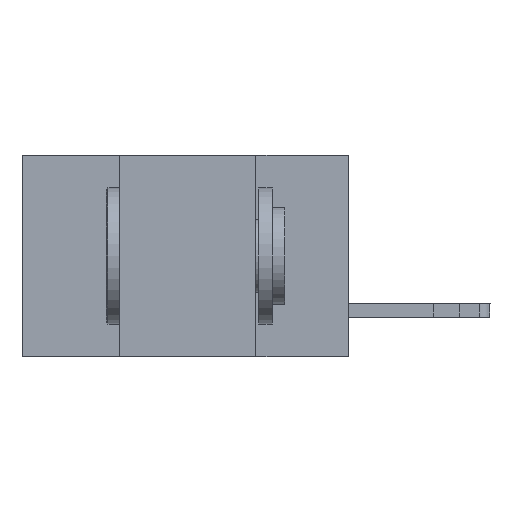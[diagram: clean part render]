
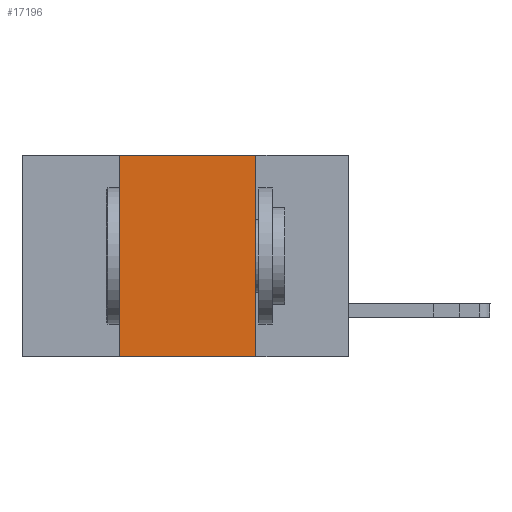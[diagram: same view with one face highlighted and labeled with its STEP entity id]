
A CAD part, left-side view. The second image highlights one B-rep face of the part: STEP entity #17196.
In plain terms, the highlighted planar face has unit normal (-1, 0, 0).
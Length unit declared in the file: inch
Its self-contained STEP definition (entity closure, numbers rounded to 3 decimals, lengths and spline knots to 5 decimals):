
#96 = CARTESIAN_POINT ( 'NONE',  ( 0., 0.6, -0.37 ) ) ;
#472 = CARTESIAN_POINT ( 'NONE',  ( 0., 0.42, -0.37 ) ) ;
#1150 = ORIENTED_EDGE ( 'NONE', *, *, #3767, .F. ) ;
#1240 = DIRECTION ( 'NONE',  ( 0., 0., 1. ) ) ;
#1275 = DIRECTION ( 'NONE',  ( 0., 0., -1. ) ) ;
#2081 = VERTEX_POINT ( 'NONE', #8609 ) ;
#2252 = ORIENTED_EDGE ( 'NONE', *, *, #8437, .F. ) ;
#2761 = CARTESIAN_POINT ( 'NONE',  ( 0., 0.42, -0.37 ) ) ;
#2810 = DIRECTION ( 'NONE',  ( 0., -1., 0. ) ) ;
#2941 = ORIENTED_EDGE ( 'NONE', *, *, #15125, .T. ) ;
#3767 = EDGE_CURVE ( 'NONE', #4106, #5642, #17734, .T. ) ;
#4106 = VERTEX_POINT ( 'NONE', #2761 ) ;
#4689 = EDGE_CURVE ( 'NONE', #5642, #8447, #13303, .T. ) ;
#5642 = VERTEX_POINT ( 'NONE', #7934 ) ;
#5670 = EDGE_LOOP ( 'NONE', ( #2252, #6712, #1150, #2941 ) ) ;
#6530 = LINE ( 'NONE', #96, #13383 ) ;
#6712 = ORIENTED_EDGE ( 'NONE', *, *, #4689, .F. ) ;
#7934 = CARTESIAN_POINT ( 'NONE',  ( 0., 0.42, 0. ) ) ;
#8136 = DIRECTION ( 'NONE',  ( 1., 0., 0. ) ) ;
#8437 = EDGE_CURVE ( 'NONE', #8447, #2081, #11788, .T. ) ;
#8447 = VERTEX_POINT ( 'NONE', #16274 ) ;
#8609 = CARTESIAN_POINT ( 'NONE',  ( 0., 0.17, -0.37 ) ) ;
#9552 = CARTESIAN_POINT ( 'NONE',  ( 0., 0.17, -0.37 ) ) ;
#11788 = LINE ( 'NONE', #9552, #14963 ) ;
#12199 = PLANE ( 'NONE',  #15303 ) ;
#12934 = FACE_OUTER_BOUND ( 'NONE', #5670, .T. ) ;
#13303 = LINE ( 'NONE', #13330, #16847 ) ;
#13330 = CARTESIAN_POINT ( 'NONE',  ( 0., 0.6, 0. ) ) ;
#13383 = VECTOR ( 'NONE', #2810, 39.37008 ) ;
#13560 = CARTESIAN_POINT ( 'NONE',  ( 0., 0.6, 0. ) ) ;
#13725 = DIRECTION ( 'NONE',  ( 0., -1., 0. ) ) ;
#14963 = VECTOR ( 'NONE', #1275, 39.37008 ) ;
#15125 = EDGE_CURVE ( 'NONE', #4106, #2081, #6530, .T. ) ;
#15303 = AXIS2_PLACEMENT_3D ( 'NONE', #13560, #8136, #17587 ) ;
#16274 = CARTESIAN_POINT ( 'NONE',  ( 0., 0.17, 0. ) ) ;
#16847 = VECTOR ( 'NONE', #13725, 39.37008 ) ;
#17196 = ADVANCED_FACE ( 'NONE', ( #12934 ), #12199, .F. ) ;
#17308 = VECTOR ( 'NONE', #1240, 39.37008 ) ;
#17587 = DIRECTION ( 'NONE',  ( 0., 0., -1. ) ) ;
#17734 = LINE ( 'NONE', #472, #17308 ) ;
